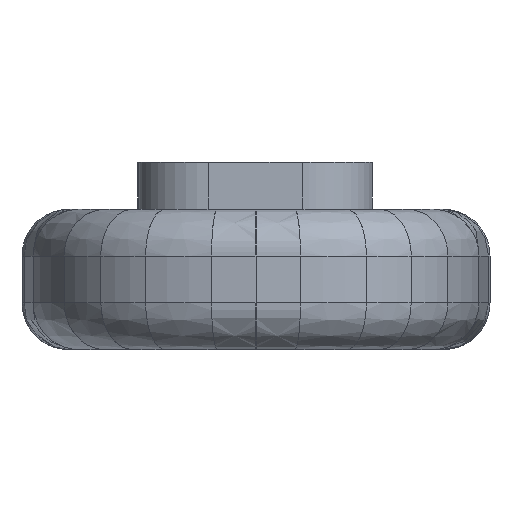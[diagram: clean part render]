
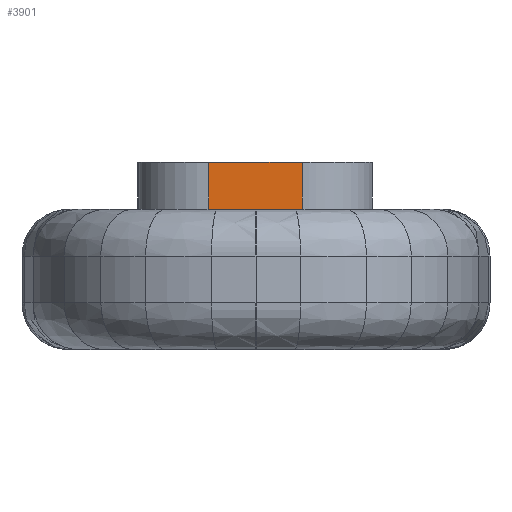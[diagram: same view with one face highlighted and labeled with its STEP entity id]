
A CAD part, left-side view. The second image highlights one B-rep face of the part: STEP entity #3901.
In plain terms, the highlighted free-form (B-spline) face has degree [1, 1] with [2, 2] control points.
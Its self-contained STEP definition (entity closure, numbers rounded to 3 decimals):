
#94 = PLANE('',#95);
#95 = AXIS2_PLACEMENT_3D('',#96,#97,#98);
#96 = CARTESIAN_POINT('',(149.225,2.54,7.62));
#97 = DIRECTION('',(0.,0.,-1.));
#98 = DIRECTION('',(-1.,0.,0.));
#336 = VERTEX_POINT('',#337);
#337 = CARTESIAN_POINT('',(85.12,15.272,7.62));
#351 = ( BOUNDED_SURFACE() B_SPLINE_SURFACE(2,1,(
    (#352,#353)
    ,(#354,#355)
,(#356,#357
    )),.UNSPECIFIED.,.F.,.F.,.F.) B_SPLINE_SURFACE_WITH_KNOTS((3,3),(2,2
    ),(0.,1.),(0.,1.),.PIECEWISE_BEZIER_KNOTS.) 
GEOMETRIC_REPRESENTATION_ITEM() RATIONAL_B_SPLINE_SURFACE((
    (1.,1.)
    ,(0.707,0.707)
,(1.,1.))) REPRESENTATION_ITEM('') SURFACE() );
#352 = CARTESIAN_POINT('',(85.12,15.272,10.16));
#353 = CARTESIAN_POINT('',(85.12,15.272,7.62));
#354 = CARTESIAN_POINT('',(85.12,19.082,10.16));
#355 = CARTESIAN_POINT('',(85.12,19.082,7.62));
#356 = CARTESIAN_POINT('',(88.93,19.082,10.16));
#357 = CARTESIAN_POINT('',(88.93,19.082,7.62));
#365 = EDGE_CURVE('',#366,#336,#368,.T.);
#366 = VERTEX_POINT('',#367);
#367 = CARTESIAN_POINT('',(85.12,10.192,7.62));
#368 = SURFACE_CURVE('',#369,(#372,#378),.PCURVE_S1.);
#369 = B_SPLINE_CURVE_WITH_KNOTS('',1,(#370,#371),.UNSPECIFIED.,.F.,.F.,
  (2,2),(0.,1.),.PIECEWISE_BEZIER_KNOTS.);
#370 = CARTESIAN_POINT('',(85.12,10.192,7.62));
#371 = CARTESIAN_POINT('',(85.12,15.272,7.62));
#372 = PCURVE('',#94,#373);
#373 = DEFINITIONAL_REPRESENTATION('',(#374),#377);
#374 = B_SPLINE_CURVE_WITH_KNOTS('',1,(#375,#376),.UNSPECIFIED.,.F.,.F.,
  (2,2),(0.,1.),.PIECEWISE_BEZIER_KNOTS.);
#375 = CARTESIAN_POINT('',(64.105,7.652));
#376 = CARTESIAN_POINT('',(64.105,12.732));
#377 = ( GEOMETRIC_REPRESENTATION_CONTEXT(2) 
PARAMETRIC_REPRESENTATION_CONTEXT() REPRESENTATION_CONTEXT('2D SPACE',''
  ) );
#378 = PCURVE('',#379,#384);
#379 = B_SPLINE_SURFACE_WITH_KNOTS('',1,1,(
    (#380,#381)
    ,(#382,#383
    )),.UNSPECIFIED.,.F.,.F.,.F.,(2,2),(2,2),(0.,1.),(0.,1.),
  .PIECEWISE_BEZIER_KNOTS.);
#380 = CARTESIAN_POINT('',(85.12,10.192,10.16));
#381 = CARTESIAN_POINT('',(85.12,10.192,7.62));
#382 = CARTESIAN_POINT('',(85.12,15.272,10.16));
#383 = CARTESIAN_POINT('',(85.12,15.272,7.62));
#384 = DEFINITIONAL_REPRESENTATION('',(#385),#389);
#385 = LINE('',#386,#387);
#386 = CARTESIAN_POINT('',(0.,1.));
#387 = VECTOR('',#388,1.);
#388 = DIRECTION('',(1.,0.));
#389 = ( GEOMETRIC_REPRESENTATION_CONTEXT(2) 
PARAMETRIC_REPRESENTATION_CONTEXT() REPRESENTATION_CONTEXT('2D SPACE',''
  ) );
#407 = ( BOUNDED_SURFACE() B_SPLINE_SURFACE(2,1,(
    (#408,#409)
    ,(#410,#411)
,(#412,#413
    )),.UNSPECIFIED.,.F.,.F.,.F.) B_SPLINE_SURFACE_WITH_KNOTS((3,3),(2,2
    ),(0.,1.),(0.,1.),.PIECEWISE_BEZIER_KNOTS.) 
GEOMETRIC_REPRESENTATION_ITEM() RATIONAL_B_SPLINE_SURFACE((
    (1.,1.)
    ,(0.707,0.707)
,(1.,1.))) REPRESENTATION_ITEM('') SURFACE() );
#408 = CARTESIAN_POINT('',(88.93,6.382,10.16));
#409 = CARTESIAN_POINT('',(88.93,6.382,7.62));
#410 = CARTESIAN_POINT('',(85.12,6.382,10.16));
#411 = CARTESIAN_POINT('',(85.12,6.382,7.62));
#412 = CARTESIAN_POINT('',(85.12,10.192,10.16));
#413 = CARTESIAN_POINT('',(85.12,10.192,7.62));
#3586 = PLANE('',#3587);
#3587 = AXIS2_PLACEMENT_3D('',#3588,#3589,#3590);
#3588 = CARTESIAN_POINT('',(92.74,17.812,10.16));
#3589 = DIRECTION('',(0.,0.,1.));
#3590 = DIRECTION('',(1.,0.,0.));
#3809 = EDGE_CURVE('',#3810,#336,#3812,.T.);
#3810 = VERTEX_POINT('',#3811);
#3811 = CARTESIAN_POINT('',(85.12,15.272,10.16));
#3812 = SURFACE_CURVE('',#3813,(#3816,#3823),.PCURVE_S1.);
#3813 = B_SPLINE_CURVE_WITH_KNOTS('',1,(#3814,#3815),.UNSPECIFIED.,.F.,
  .F.,(2,2),(0.,1.),.PIECEWISE_BEZIER_KNOTS.);
#3814 = CARTESIAN_POINT('',(85.12,15.272,10.16));
#3815 = CARTESIAN_POINT('',(85.12,15.272,7.62));
#3816 = PCURVE('',#351,#3817);
#3817 = DEFINITIONAL_REPRESENTATION('',(#3818),#3822);
#3818 = LINE('',#3819,#3820);
#3819 = CARTESIAN_POINT('',(0.,0.));
#3820 = VECTOR('',#3821,1.);
#3821 = DIRECTION('',(0.,1.));
#3822 = ( GEOMETRIC_REPRESENTATION_CONTEXT(2) 
PARAMETRIC_REPRESENTATION_CONTEXT() REPRESENTATION_CONTEXT('2D SPACE',''
  ) );
#3823 = PCURVE('',#379,#3824);
#3824 = DEFINITIONAL_REPRESENTATION('',(#3825),#3829);
#3825 = LINE('',#3826,#3827);
#3826 = CARTESIAN_POINT('',(1.,0.));
#3827 = VECTOR('',#3828,1.);
#3828 = DIRECTION('',(0.,1.));
#3829 = ( GEOMETRIC_REPRESENTATION_CONTEXT(2) 
PARAMETRIC_REPRESENTATION_CONTEXT() REPRESENTATION_CONTEXT('2D SPACE',''
  ) );
#3859 = VERTEX_POINT('',#3860);
#3860 = CARTESIAN_POINT('',(85.12,10.192,10.16));
#3881 = EDGE_CURVE('',#3859,#366,#3882,.T.);
#3882 = SURFACE_CURVE('',#3883,(#3886,#3893),.PCURVE_S1.);
#3883 = B_SPLINE_CURVE_WITH_KNOTS('',1,(#3884,#3885),.UNSPECIFIED.,.F.,
  .F.,(2,2),(0.,1.),.PIECEWISE_BEZIER_KNOTS.);
#3884 = CARTESIAN_POINT('',(85.12,10.192,10.16));
#3885 = CARTESIAN_POINT('',(85.12,10.192,7.62));
#3886 = PCURVE('',#407,#3887);
#3887 = DEFINITIONAL_REPRESENTATION('',(#3888),#3892);
#3888 = LINE('',#3889,#3890);
#3889 = CARTESIAN_POINT('',(1.,0.));
#3890 = VECTOR('',#3891,1.);
#3891 = DIRECTION('',(0.,1.));
#3892 = ( GEOMETRIC_REPRESENTATION_CONTEXT(2) 
PARAMETRIC_REPRESENTATION_CONTEXT() REPRESENTATION_CONTEXT('2D SPACE',''
  ) );
#3893 = PCURVE('',#379,#3894);
#3894 = DEFINITIONAL_REPRESENTATION('',(#3895),#3899);
#3895 = LINE('',#3896,#3897);
#3896 = CARTESIAN_POINT('',(0.,0.));
#3897 = VECTOR('',#3898,1.);
#3898 = DIRECTION('',(0.,1.));
#3899 = ( GEOMETRIC_REPRESENTATION_CONTEXT(2) 
PARAMETRIC_REPRESENTATION_CONTEXT() REPRESENTATION_CONTEXT('2D SPACE',''
  ) );
#3901 = ADVANCED_FACE('',(#3902),#379,.T.);
#3902 = FACE_BOUND('',#3903,.T.);
#3903 = EDGE_LOOP('',(#3904,#3905,#3924,#3925));
#3904 = ORIENTED_EDGE('',*,*,#3881,.F.);
#3905 = ORIENTED_EDGE('',*,*,#3906,.T.);
#3906 = EDGE_CURVE('',#3859,#3810,#3907,.T.);
#3907 = SURFACE_CURVE('',#3908,(#3911,#3918),.PCURVE_S1.);
#3908 = B_SPLINE_CURVE_WITH_KNOTS('',1,(#3909,#3910),.UNSPECIFIED.,.F.,
  .F.,(2,2),(0.,1.),.PIECEWISE_BEZIER_KNOTS.);
#3909 = CARTESIAN_POINT('',(85.12,10.192,10.16));
#3910 = CARTESIAN_POINT('',(85.12,15.272,10.16));
#3911 = PCURVE('',#379,#3912);
#3912 = DEFINITIONAL_REPRESENTATION('',(#3913),#3917);
#3913 = LINE('',#3914,#3915);
#3914 = CARTESIAN_POINT('',(0.,0.));
#3915 = VECTOR('',#3916,1.);
#3916 = DIRECTION('',(1.,0.));
#3917 = ( GEOMETRIC_REPRESENTATION_CONTEXT(2) 
PARAMETRIC_REPRESENTATION_CONTEXT() REPRESENTATION_CONTEXT('2D SPACE',''
  ) );
#3918 = PCURVE('',#3586,#3919);
#3919 = DEFINITIONAL_REPRESENTATION('',(#3920),#3923);
#3920 = B_SPLINE_CURVE_WITH_KNOTS('',1,(#3921,#3922),.UNSPECIFIED.,.F.,
  .F.,(2,2),(0.,1.),.PIECEWISE_BEZIER_KNOTS.);
#3921 = CARTESIAN_POINT('',(-7.62,-7.62));
#3922 = CARTESIAN_POINT('',(-7.62,-2.54));
#3923 = ( GEOMETRIC_REPRESENTATION_CONTEXT(2) 
PARAMETRIC_REPRESENTATION_CONTEXT() REPRESENTATION_CONTEXT('2D SPACE',''
  ) );
#3924 = ORIENTED_EDGE('',*,*,#3809,.T.);
#3925 = ORIENTED_EDGE('',*,*,#365,.F.);
